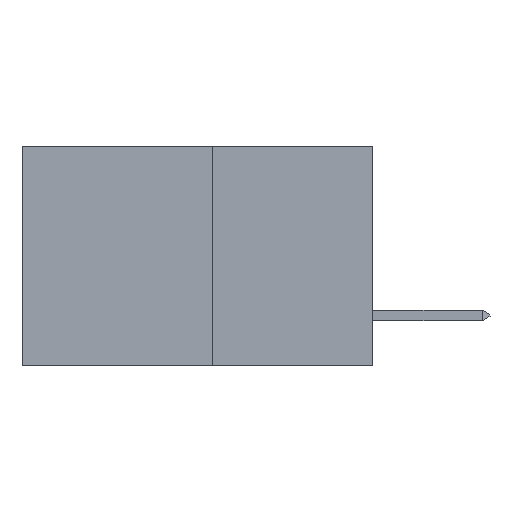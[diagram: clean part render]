
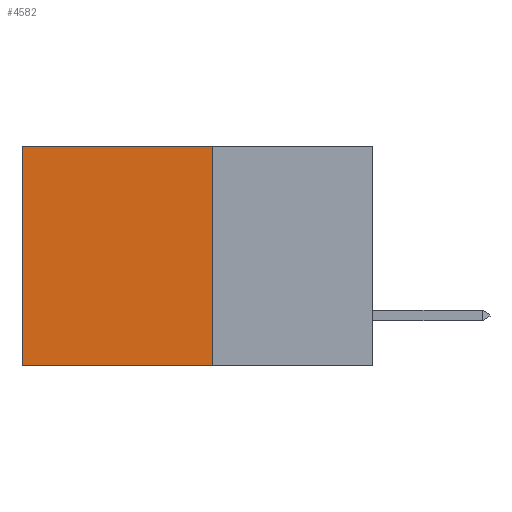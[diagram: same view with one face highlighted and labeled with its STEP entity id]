
A CAD part, left-side view. The second image highlights one B-rep face of the part: STEP entity #4582.
In plain terms, the highlighted planar face has unit normal (-1, 0, 0).
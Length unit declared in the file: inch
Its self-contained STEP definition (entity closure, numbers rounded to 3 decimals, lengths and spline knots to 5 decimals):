
#275 = VECTOR ( 'NONE', #2710, 39.37008 ) ;
#716 = DIRECTION ( 'NONE',  ( 1., 0., 0. ) ) ;
#759 = EDGE_CURVE ( 'NONE', #5398, #3266, #5366, .T. ) ;
#802 = CARTESIAN_POINT ( 'NONE',  ( 0.277, 0.59, 0. ) ) ;
#822 = LINE ( 'NONE', #1849, #8136 ) ;
#1337 = DIRECTION ( 'NONE',  ( 0., 0., -1. ) ) ;
#1651 = CARTESIAN_POINT ( 'NONE',  ( 0.277, 0.27, -0.37 ) ) ;
#1653 = ORIENTED_EDGE ( 'NONE', *, *, #759, .F. ) ;
#1705 = CARTESIAN_POINT ( 'NONE',  ( 0.277, 0.59, -0.37 ) ) ;
#1706 = VERTEX_POINT ( 'NONE', #6277 ) ;
#1849 = CARTESIAN_POINT ( 'NONE',  ( 0.277, 0.27, -0.37 ) ) ;
#2114 = LINE ( 'NONE', #4891, #275 ) ;
#2325 = PLANE ( 'NONE',  #5440 ) ;
#2578 = DIRECTION ( 'NONE',  ( 0., 1., 0. ) ) ;
#2668 = CARTESIAN_POINT ( 'NONE',  ( 0.277, 0.27, -0.37 ) ) ;
#2710 = DIRECTION ( 'NONE',  ( 0., 1., 0. ) ) ;
#3266 = VERTEX_POINT ( 'NONE', #1705 ) ;
#3349 = EDGE_CURVE ( 'NONE', #4686, #3266, #7801, .T. ) ;
#3359 = DIRECTION ( 'NONE',  ( 0., 0., -1. ) ) ;
#4582 = ADVANCED_FACE ( 'NONE', ( #6551 ), #2325, .F. ) ;
#4591 = DIRECTION ( 'NONE',  ( 0., 0., -1. ) ) ;
#4686 = VERTEX_POINT ( 'NONE', #802 ) ;
#4891 = CARTESIAN_POINT ( 'NONE',  ( 0.277, 0.27, 0. ) ) ;
#4926 = ORIENTED_EDGE ( 'NONE', *, *, #7643, .T. ) ;
#5366 = LINE ( 'NONE', #8205, #6995 ) ;
#5398 = VERTEX_POINT ( 'NONE', #2668 ) ;
#5440 = AXIS2_PLACEMENT_3D ( 'NONE', #1651, #716, #4591 ) ;
#5455 = ORIENTED_EDGE ( 'NONE', *, *, #6931, .F. ) ;
#5941 = VECTOR ( 'NONE', #1337, 39.37008 ) ;
#6087 = CARTESIAN_POINT ( 'NONE',  ( 0.277, 0.59, -0.37 ) ) ;
#6277 = CARTESIAN_POINT ( 'NONE',  ( 0.277, 0.27, 0. ) ) ;
#6551 = FACE_OUTER_BOUND ( 'NONE', #8744, .T. ) ;
#6931 = EDGE_CURVE ( 'NONE', #1706, #5398, #822, .T. ) ;
#6995 = VECTOR ( 'NONE', #2578, 39.37008 ) ;
#7643 = EDGE_CURVE ( 'NONE', #1706, #4686, #2114, .T. ) ;
#7801 = LINE ( 'NONE', #6087, #5941 ) ;
#8136 = VECTOR ( 'NONE', #3359, 39.37008 ) ;
#8205 = CARTESIAN_POINT ( 'NONE',  ( 0.277, 0.27, -0.37 ) ) ;
#8744 = EDGE_LOOP ( 'NONE', ( #8938, #1653, #5455, #4926 ) ) ;
#8938 = ORIENTED_EDGE ( 'NONE', *, *, #3349, .T. ) ;
